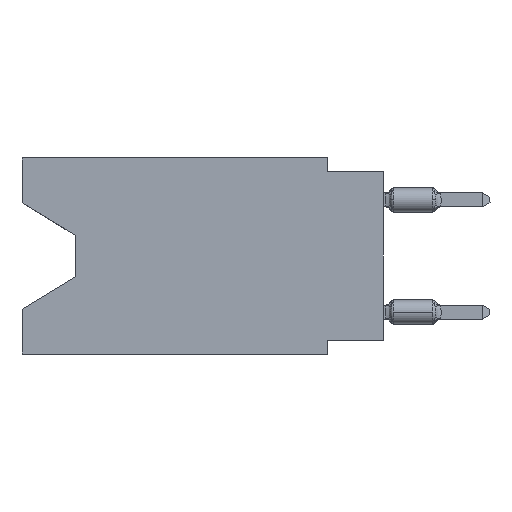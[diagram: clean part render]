
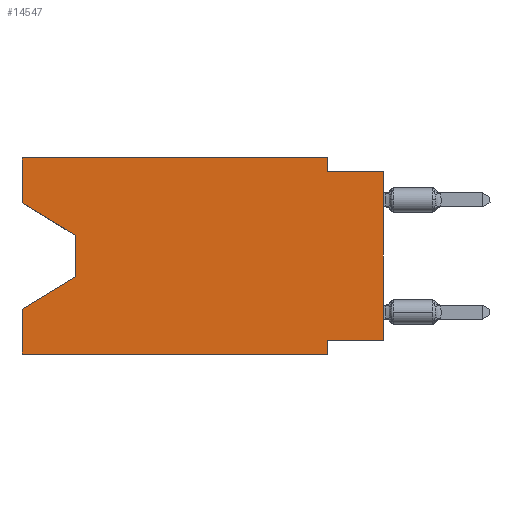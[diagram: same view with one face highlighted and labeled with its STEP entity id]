
A CAD part, left-side view. The second image highlights one B-rep face of the part: STEP entity #14547.
In plain terms, the highlighted planar face has unit normal (-1, 0, 0).
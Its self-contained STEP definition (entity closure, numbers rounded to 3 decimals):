
#465 = CARTESIAN_POINT ( 'NONE',  ( 0., 0., -8.255 ) ) ;
#896 = CARTESIAN_POINT ( 'NONE',  ( 0., 16.383, 0. ) ) ;
#987 = VECTOR ( 'NONE', #7394, 1000. ) ;
#1241 = DIRECTION ( 'NONE',  ( 0., -1., 0. ) ) ;
#1272 = AXIS2_PLACEMENT_3D ( 'NONE', #7136, #3877, #15233 ) ;
#1340 = ORIENTED_EDGE ( 'NONE', *, *, #10765, .F. ) ;
#1445 = VERTEX_POINT ( 'NONE', #18246 ) ;
#1544 = CARTESIAN_POINT ( 'NONE',  ( 0., 13.97, -3.505 ) ) ;
#1736 = LINE ( 'NONE', #4688, #987 ) ;
#1911 = CARTESIAN_POINT ( 'NONE',  ( 0., 16.383, -2.038 ) ) ;
#2734 = ORIENTED_EDGE ( 'NONE', *, *, #13687, .F. ) ;
#3112 = VERTEX_POINT ( 'NONE', #896 ) ;
#3325 = VECTOR ( 'NONE', #1241, 1000. ) ;
#3422 = VECTOR ( 'NONE', #10090, 1000. ) ;
#3523 = VERTEX_POINT ( 'NONE', #8146 ) ;
#3525 = CARTESIAN_POINT ( 'NONE',  ( 0., 2.54, -8.89 ) ) ;
#3550 = CARTESIAN_POINT ( 'NONE',  ( 0., 0., -0.635 ) ) ;
#3877 = DIRECTION ( 'NONE',  ( 1., 0., 0. ) ) ;
#3959 = LINE ( 'NONE', #16515, #11024 ) ;
#3961 = CARTESIAN_POINT ( 'NONE',  ( 0., 0., -0.635 ) ) ;
#4001 = ORIENTED_EDGE ( 'NONE', *, *, #9905, .F. ) ;
#4288 = LINE ( 'NONE', #12932, #13489 ) ;
#4330 = LINE ( 'NONE', #10006, #3422 ) ;
#4461 = CARTESIAN_POINT ( 'NONE',  ( 0., 16.383, 0. ) ) ;
#4631 = VECTOR ( 'NONE', #9713, 1000. ) ;
#4639 = DIRECTION ( 'NONE',  ( 0., 0., 1. ) ) ;
#4688 = CARTESIAN_POINT ( 'NONE',  ( 0., 16.383, 0. ) ) ;
#4836 = EDGE_CURVE ( 'NONE', #6521, #3112, #1736, .T. ) ;
#4948 = ORIENTED_EDGE ( 'NONE', *, *, #14130, .T. ) ;
#5327 = LINE ( 'NONE', #12400, #4631 ) ;
#5397 = DIRECTION ( 'NONE',  ( 0., 0., -1. ) ) ;
#5451 = CARTESIAN_POINT ( 'NONE',  ( 0., 16.383, -2.038 ) ) ;
#5868 = EDGE_CURVE ( 'NONE', #6521, #9456, #18196, .T. ) ;
#5992 = VECTOR ( 'NONE', #17784, 1000. ) ;
#6323 = EDGE_CURVE ( 'NONE', #7573, #16009, #5327, .T. ) ;
#6350 = DIRECTION ( 'NONE',  ( 0., 1., 0. ) ) ;
#6521 = VERTEX_POINT ( 'NONE', #1911 ) ;
#7092 = EDGE_CURVE ( 'NONE', #3112, #13649, #10244, .T. ) ;
#7136 = CARTESIAN_POINT ( 'NONE',  ( 0., 16.383, 0. ) ) ;
#7202 = ORIENTED_EDGE ( 'NONE', *, *, #7092, .F. ) ;
#7246 = VECTOR ( 'NONE', #6350, 1000. ) ;
#7394 = DIRECTION ( 'NONE',  ( 0., 0., 1. ) ) ;
#7538 = ORIENTED_EDGE ( 'NONE', *, *, #6323, .T. ) ;
#7573 = VERTEX_POINT ( 'NONE', #465 ) ;
#7716 = ORIENTED_EDGE ( 'NONE', *, *, #5868, .T. ) ;
#7951 = VECTOR ( 'NONE', #15646, 1000. ) ;
#8146 = CARTESIAN_POINT ( 'NONE',  ( 0., 2.54, -0.635 ) ) ;
#9056 = VERTEX_POINT ( 'NONE', #10016 ) ;
#9092 = VECTOR ( 'NONE', #9734, 1000. ) ;
#9456 = VERTEX_POINT ( 'NONE', #1544 ) ;
#9527 = CARTESIAN_POINT ( 'NONE',  ( 0., 2.54, 0. ) ) ;
#9652 = PLANE ( 'NONE',  #1272 ) ;
#9713 = DIRECTION ( 'NONE',  ( 0., 0., 1. ) ) ;
#9734 = DIRECTION ( 'NONE',  ( 0., -0.855, -0.519 ) ) ;
#9905 = EDGE_CURVE ( 'NONE', #13321, #9056, #17028, .T. ) ;
#10006 = CARTESIAN_POINT ( 'NONE',  ( 0., 13.97, -3.505 ) ) ;
#10016 = CARTESIAN_POINT ( 'NONE',  ( 0., 16.383, -6.852 ) ) ;
#10040 = CARTESIAN_POINT ( 'NONE',  ( 0., 16.383, 0. ) ) ;
#10090 = DIRECTION ( 'NONE',  ( 0., 0., -1. ) ) ;
#10174 = VECTOR ( 'NONE', #4639, 1000. ) ;
#10244 = LINE ( 'NONE', #4461, #7951 ) ;
#10258 = LINE ( 'NONE', #13044, #7246 ) ;
#10547 = ORIENTED_EDGE ( 'NONE', *, *, #4836, .F. ) ;
#10765 = EDGE_CURVE ( 'NONE', #3523, #16009, #16298, .T. ) ;
#10804 = VECTOR ( 'NONE', #5397, 1000. ) ;
#10988 = CARTESIAN_POINT ( 'NONE',  ( 0., 16.383, -8.89 ) ) ;
#11024 = VECTOR ( 'NONE', #16792, 1000. ) ;
#11424 = FACE_OUTER_BOUND ( 'NONE', #12019, .T. ) ;
#12019 = EDGE_LOOP ( 'NONE', ( #7716, #12112, #17900, #4001, #4948, #17190, #17231, #7538, #1340, #2734, #7202, #10547 ) ) ;
#12112 = ORIENTED_EDGE ( 'NONE', *, *, #16183, .T. ) ;
#12400 = CARTESIAN_POINT ( 'NONE',  ( 0., 0., 0. ) ) ;
#12657 = CARTESIAN_POINT ( 'NONE',  ( 0., 2.54, -8.89 ) ) ;
#12932 = CARTESIAN_POINT ( 'NONE',  ( 0., 13.97, -5.385 ) ) ;
#13044 = CARTESIAN_POINT ( 'NONE',  ( 0., 0., -8.255 ) ) ;
#13321 = VERTEX_POINT ( 'NONE', #13740 ) ;
#13489 = VECTOR ( 'NONE', #17122, 1000. ) ;
#13517 = CARTESIAN_POINT ( 'NONE',  ( 0., 2.54, -8.255 ) ) ;
#13649 = VERTEX_POINT ( 'NONE', #9527 ) ;
#13687 = EDGE_CURVE ( 'NONE', #13649, #3523, #3959, .T. ) ;
#13740 = CARTESIAN_POINT ( 'NONE',  ( 0., 16.383, -8.89 ) ) ;
#14066 = VERTEX_POINT ( 'NONE', #13517 ) ;
#14130 = EDGE_CURVE ( 'NONE', #13321, #15401, #15087, .T. ) ;
#14547 = ADVANCED_FACE ( 'NONE', ( #11424 ), #9652, .F. ) ;
#15087 = LINE ( 'NONE', #10988, #3325 ) ;
#15233 = DIRECTION ( 'NONE',  ( 0., 0., -1. ) ) ;
#15258 = EDGE_CURVE ( 'NONE', #1445, #9056, #4288, .T. ) ;
#15401 = VERTEX_POINT ( 'NONE', #3525 ) ;
#15646 = DIRECTION ( 'NONE',  ( 0., -1., 0. ) ) ;
#16009 = VERTEX_POINT ( 'NONE', #3961 ) ;
#16183 = EDGE_CURVE ( 'NONE', #9456, #1445, #4330, .T. ) ;
#16298 = LINE ( 'NONE', #3550, #5992 ) ;
#16515 = CARTESIAN_POINT ( 'NONE',  ( 0., 2.54, 0. ) ) ;
#16792 = DIRECTION ( 'NONE',  ( 0., 0., -1. ) ) ;
#16929 = LINE ( 'NONE', #12657, #10804 ) ;
#17028 = LINE ( 'NONE', #10040, #10174 ) ;
#17122 = DIRECTION ( 'NONE',  ( 0., 0.855, -0.519 ) ) ;
#17190 = ORIENTED_EDGE ( 'NONE', *, *, #18044, .F. ) ;
#17231 = ORIENTED_EDGE ( 'NONE', *, *, #17849, .F. ) ;
#17784 = DIRECTION ( 'NONE',  ( 0., -1., 0. ) ) ;
#17849 = EDGE_CURVE ( 'NONE', #7573, #14066, #10258, .T. ) ;
#17900 = ORIENTED_EDGE ( 'NONE', *, *, #15258, .T. ) ;
#18044 = EDGE_CURVE ( 'NONE', #14066, #15401, #16929, .T. ) ;
#18196 = LINE ( 'NONE', #5451, #9092 ) ;
#18246 = CARTESIAN_POINT ( 'NONE',  ( 0., 13.97, -5.385 ) ) ;
